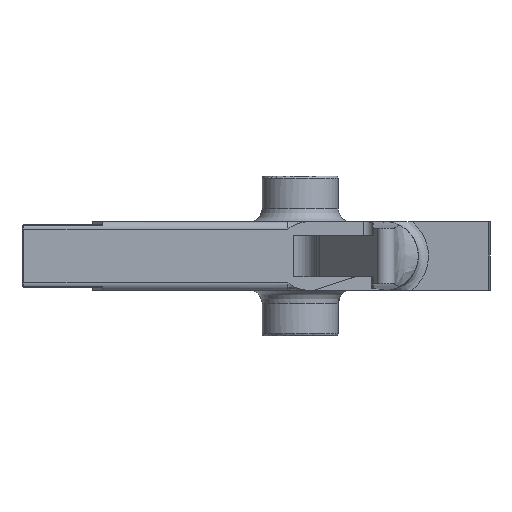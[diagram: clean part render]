
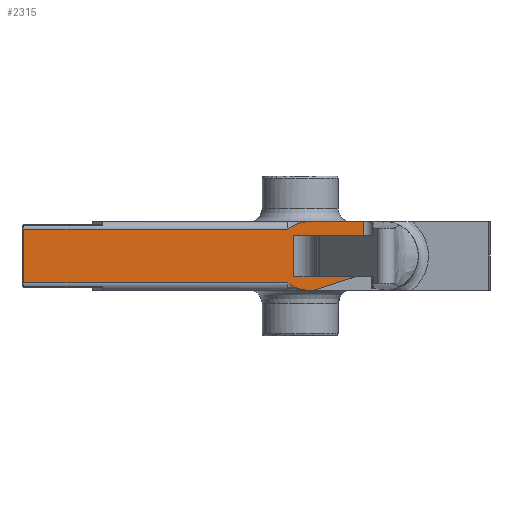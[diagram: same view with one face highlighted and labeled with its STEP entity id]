
A CAD part, front view. The second image highlights one B-rep face of the part: STEP entity #2315.
In plain terms, the highlighted planar face has unit normal (0, -1, 0).
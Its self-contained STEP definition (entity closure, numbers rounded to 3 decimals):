
#52=B_SPLINE_CURVE_WITH_KNOTS('',3,(#3445,#3446,#3447,#3448,#3449,#3450,
#3451,#3452),.UNSPECIFIED.,.F.,.F.,(4,2,2,4),(-0.236,-0.229,
-0.139,-0.073),.UNSPECIFIED.);
#53=B_SPLINE_CURVE_WITH_KNOTS('',3,(#3460,#3461,#3462,#3463,#3464,#3465,
#3466,#3467),.UNSPECIFIED.,.F.,.F.,(4,2,2,4),(-0.183,-0.106,
0.,0.008),.UNSPECIFIED.);
#146=PLANE('',#2472);
#197=FACE_OUTER_BOUND('',#330,.T.);
#330=EDGE_LOOP('',(#1552,#1553,#1554,#1555,#1556,#1557,#1558,#1559,#1560,
#1561,#1562,#1563,#1564,#1565));
#461=LINE('',#3396,#631);
#473=LINE('',#3429,#643);
#474=LINE('',#3434,#644);
#475=LINE('',#3437,#645);
#476=LINE('',#3439,#646);
#477=LINE('',#3441,#647);
#478=LINE('',#3443,#648);
#479=LINE('',#3454,#649);
#480=LINE('',#3456,#650);
#481=LINE('',#3458,#651);
#482=LINE('',#3469,#652);
#483=LINE('',#3470,#653);
#631=VECTOR('',#2721,10.);
#643=VECTOR('',#2751,10.);
#644=VECTOR('',#2756,10.);
#645=VECTOR('',#2761,10.);
#646=VECTOR('',#2762,10.);
#647=VECTOR('',#2763,10.);
#648=VECTOR('',#2764,10.);
#649=VECTOR('',#2765,28.619);
#650=VECTOR('',#2766,10.);
#651=VECTOR('',#2767,28.619);
#652=VECTOR('',#2768,10.);
#653=VECTOR('',#2769,10.);
#913=VERTEX_POINT('',#3393);
#914=VERTEX_POINT('',#3395);
#926=VERTEX_POINT('',#3427);
#927=VERTEX_POINT('',#3431);
#928=VERTEX_POINT('',#3433);
#929=VERTEX_POINT('',#3438);
#930=VERTEX_POINT('',#3440);
#931=VERTEX_POINT('',#3442);
#932=VERTEX_POINT('',#3444);
#933=VERTEX_POINT('',#3453);
#934=VERTEX_POINT('',#3455);
#935=VERTEX_POINT('',#3457);
#936=VERTEX_POINT('',#3459);
#937=VERTEX_POINT('',#3468);
#1150=EDGE_CURVE('',#914,#913,#461,.T.);
#1167=EDGE_CURVE('',#926,#913,#473,.T.);
#1169=EDGE_CURVE('',#927,#928,#474,.T.);
#1171=EDGE_CURVE('',#926,#928,#475,.T.);
#1172=EDGE_CURVE('',#929,#927,#476,.T.);
#1173=EDGE_CURVE('',#930,#929,#477,.T.);
#1174=EDGE_CURVE('',#931,#930,#478,.T.);
#1175=EDGE_CURVE('',#932,#931,#52,.T.);
#1176=EDGE_CURVE('',#932,#933,#479,.T.);
#1177=EDGE_CURVE('',#934,#933,#480,.T.);
#1178=EDGE_CURVE('',#934,#935,#481,.T.);
#1179=EDGE_CURVE('',#936,#935,#53,.T.);
#1180=EDGE_CURVE('',#937,#936,#482,.T.);
#1181=EDGE_CURVE('',#914,#937,#483,.T.);
#1552=ORIENTED_EDGE('',*,*,#1171,.T.);
#1553=ORIENTED_EDGE('',*,*,#1169,.F.);
#1554=ORIENTED_EDGE('',*,*,#1172,.F.);
#1555=ORIENTED_EDGE('',*,*,#1173,.F.);
#1556=ORIENTED_EDGE('',*,*,#1174,.F.);
#1557=ORIENTED_EDGE('',*,*,#1175,.F.);
#1558=ORIENTED_EDGE('',*,*,#1176,.T.);
#1559=ORIENTED_EDGE('',*,*,#1177,.F.);
#1560=ORIENTED_EDGE('',*,*,#1178,.T.);
#1561=ORIENTED_EDGE('',*,*,#1179,.F.);
#1562=ORIENTED_EDGE('',*,*,#1180,.F.);
#1563=ORIENTED_EDGE('',*,*,#1181,.F.);
#1564=ORIENTED_EDGE('',*,*,#1150,.T.);
#1565=ORIENTED_EDGE('',*,*,#1167,.F.);
#2315=ADVANCED_FACE('',(#197),#146,.T.);
#2472=AXIS2_PLACEMENT_3D('',#3436,#2759,#2760);
#2721=DIRECTION('',(-1.,0.,0.));
#2751=DIRECTION('',(0.,0.,-1.));
#2756=DIRECTION('',(0.,0.,1.));
#2759=DIRECTION('center_axis',(0.,-1.,0.));
#2760=DIRECTION('ref_axis',(0.,0.,
-1.));
#2761=DIRECTION('',(1.,0.,0.));
#2762=DIRECTION('',(-0.949,0.,-0.315));
#2763=DIRECTION('',(0.,0.,-1.));
#2764=DIRECTION('',(1.,0.,0.));
#2765=DIRECTION('',(-1.,0.,0.));
#2766=DIRECTION('',(0.,0.,1.));
#2767=DIRECTION('',(1.,0.,0.));
#2768=DIRECTION('',(-1.,0.,0.));
#2769=DIRECTION('',(-0.949,0.,-0.315));
#3393=CARTESIAN_POINT('',(37.042,128.537,23.721));
#3395=CARTESIAN_POINT('',(43.583,128.537,23.721));
#3396=CARTESIAN_POINT('',(23.272,128.537,23.721));
#3427=CARTESIAN_POINT('',(37.042,128.537,28.221));
#3429=CARTESIAN_POINT('',(37.042,128.537,25.254));
#3431=CARTESIAN_POINT('',(43.742,128.537,23.773));
#3433=CARTESIAN_POINT('',(43.742,128.537,28.221));
#3434=CARTESIAN_POINT('',(43.742,128.537,23.004));
#3436=CARTESIAN_POINT('Origin',(7.003,128.537,22.288));
#3437=CARTESIAN_POINT('',(24.122,128.537,28.221));
#3438=CARTESIAN_POINT('',(44.604,128.537,24.059));
#3439=CARTESIAN_POINT('',(45.165,128.537,24.245));
#3440=CARTESIAN_POINT('',(44.604,128.537,29.654));
#3441=CARTESIAN_POINT('',(44.604,128.537,25.629));
#3442=CARTESIAN_POINT('',(38.649,128.537,29.654));
#3443=CARTESIAN_POINT('',(40.283,128.537,29.654));
#3444=CARTESIAN_POINT('',(36.409,128.537,28.866));
#3445=CARTESIAN_POINT('Ctrl Pts',(36.409,128.537,28.866));
#3446=CARTESIAN_POINT('Ctrl Pts',(36.43,128.537,28.881));
#3447=CARTESIAN_POINT('Ctrl Pts',(36.452,128.537,28.896));
#3448=CARTESIAN_POINT('Ctrl Pts',(36.766,128.537,29.111));
#3449=CARTESIAN_POINT('Ctrl Pts',(37.163,128.537,29.346));
#3450=CARTESIAN_POINT('Ctrl Pts',(38.014,128.537,29.608));
#3451=CARTESIAN_POINT('Ctrl Pts',(38.349,128.537,29.654));
#3452=CARTESIAN_POINT('Ctrl Pts',(38.649,128.537,29.654));
#3453=CARTESIAN_POINT('',(8.06,128.537,28.866));
#3454=CARTESIAN_POINT('',(36.409,128.537,28.866));
#3455=CARTESIAN_POINT('',(8.06,128.537,23.075));
#3456=CARTESIAN_POINT('',(8.06,128.537,25.805));
#3457=CARTESIAN_POINT('',(36.409,128.537,23.075));
#3458=CARTESIAN_POINT('',(7.79,128.537,23.075));
#3459=CARTESIAN_POINT('',(38.649,128.537,22.288));
#3460=CARTESIAN_POINT('Ctrl Pts',(38.649,128.537,22.288));
#3461=CARTESIAN_POINT('Ctrl Pts',(38.349,128.537,22.288));
#3462=CARTESIAN_POINT('Ctrl Pts',(38.014,128.537,22.333));
#3463=CARTESIAN_POINT('Ctrl Pts',(37.163,128.537,22.595));
#3464=CARTESIAN_POINT('Ctrl Pts',(36.766,128.537,22.83));
#3465=CARTESIAN_POINT('Ctrl Pts',(36.452,128.537,23.045));
#3466=CARTESIAN_POINT('Ctrl Pts',(36.43,128.537,23.06));
#3467=CARTESIAN_POINT('Ctrl Pts',(36.409,128.537,23.075));
#3468=CARTESIAN_POINT('',(39.261,128.537,22.288));
#3469=CARTESIAN_POINT('',(37.073,128.537,22.288));
#3470=CARTESIAN_POINT('',(45.165,128.537,24.245));
